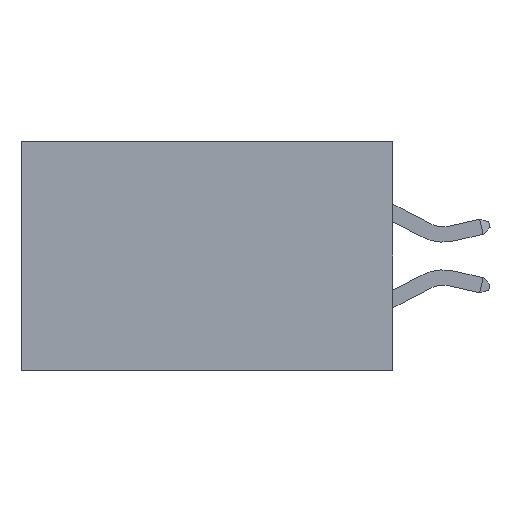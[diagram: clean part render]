
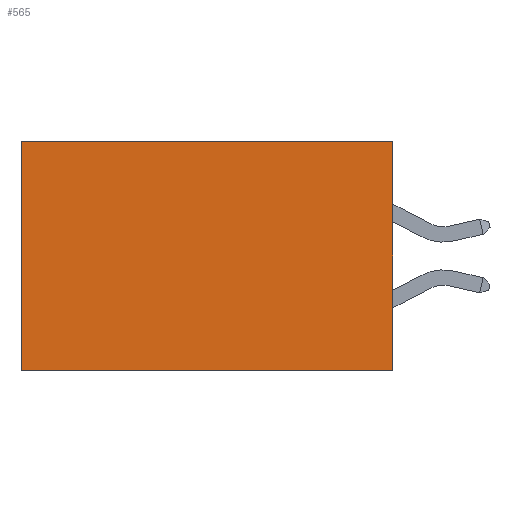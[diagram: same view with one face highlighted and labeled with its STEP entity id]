
A CAD part, left-side view. The second image highlights one B-rep face of the part: STEP entity #565.
In plain terms, the highlighted planar face has unit normal (-1, 0, 0).
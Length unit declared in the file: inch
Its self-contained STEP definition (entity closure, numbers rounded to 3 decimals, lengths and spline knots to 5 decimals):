
#104 = DIRECTION ( 'NONE',  ( 0., 1., 0. ) ) ;
#449 = LINE ( 'NONE', #13675, #2573 ) ;
#489 = EDGE_LOOP ( 'NONE', ( #5280, #5119, #11376, #10513 ) ) ;
#565 = ADVANCED_FACE ( 'NONE', ( #8681 ), #1339, .F. ) ;
#743 = CARTESIAN_POINT ( 'NONE',  ( 0.2875, 0.6, -0.37 ) ) ;
#1339 = PLANE ( 'NONE',  #12008 ) ;
#2184 = EDGE_CURVE ( 'NONE', #2218, #14663, #9671, .T. ) ;
#2218 = VERTEX_POINT ( 'NONE', #3009 ) ;
#2355 = CARTESIAN_POINT ( 'NONE',  ( 0.2875, 0.6, 0. ) ) ;
#2485 = CARTESIAN_POINT ( 'NONE',  ( 0.2875, 0., 0. ) ) ;
#2573 = VECTOR ( 'NONE', #104, 39.37008 ) ;
#2619 = CARTESIAN_POINT ( 'NONE',  ( 0.2875, 0., -0.37 ) ) ;
#2634 = EDGE_CURVE ( 'NONE', #12305, #14663, #7164, .T. ) ;
#2938 = CARTESIAN_POINT ( 'NONE',  ( 0.2875, 0., 0. ) ) ;
#3009 = CARTESIAN_POINT ( 'NONE',  ( 0.2875, 0., -0.37 ) ) ;
#4219 = LINE ( 'NONE', #2938, #9843 ) ;
#5119 = ORIENTED_EDGE ( 'NONE', *, *, #2184, .F. ) ;
#5280 = ORIENTED_EDGE ( 'NONE', *, *, #2634, .T. ) ;
#7081 = VERTEX_POINT ( 'NONE', #12091 ) ;
#7164 = LINE ( 'NONE', #7950, #12165 ) ;
#7358 = DIRECTION ( 'NONE',  ( 0., 0., -1. ) ) ;
#7950 = CARTESIAN_POINT ( 'NONE',  ( 0.2875, 0.6, 0. ) ) ;
#8341 = DIRECTION ( 'NONE',  ( 0., 1., 0. ) ) ;
#8681 = FACE_OUTER_BOUND ( 'NONE', #489, .T. ) ;
#9371 = DIRECTION ( 'NONE',  ( 0., 0., -1. ) ) ;
#9671 = LINE ( 'NONE', #2619, #13430 ) ;
#9843 = VECTOR ( 'NONE', #7358, 39.37008 ) ;
#10433 = DIRECTION ( 'NONE',  ( 1., 0., 0. ) ) ;
#10513 = ORIENTED_EDGE ( 'NONE', *, *, #14253, .T. ) ;
#11376 = ORIENTED_EDGE ( 'NONE', *, *, #14589, .F. ) ;
#12008 = AXIS2_PLACEMENT_3D ( 'NONE', #2485, #10433, #13922 ) ;
#12091 = CARTESIAN_POINT ( 'NONE',  ( 0.2875, 0., 0. ) ) ;
#12165 = VECTOR ( 'NONE', #9371, 39.37008 ) ;
#12305 = VERTEX_POINT ( 'NONE', #2355 ) ;
#13430 = VECTOR ( 'NONE', #8341, 39.37008 ) ;
#13675 = CARTESIAN_POINT ( 'NONE',  ( 0.2875, 0., 0. ) ) ;
#13922 = DIRECTION ( 'NONE',  ( 0., 0., -1. ) ) ;
#14253 = EDGE_CURVE ( 'NONE', #7081, #12305, #449, .T. ) ;
#14589 = EDGE_CURVE ( 'NONE', #7081, #2218, #4219, .T. ) ;
#14663 = VERTEX_POINT ( 'NONE', #743 ) ;
